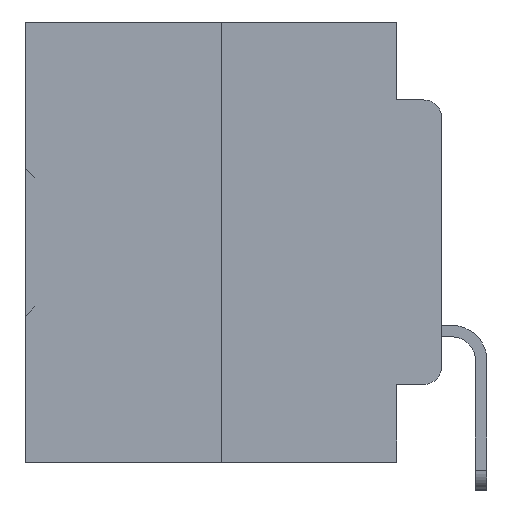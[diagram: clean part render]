
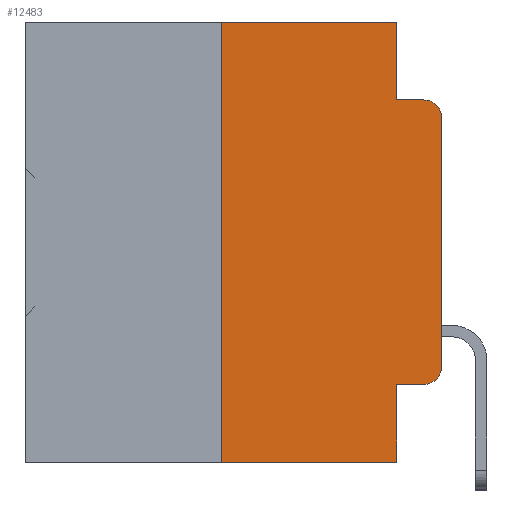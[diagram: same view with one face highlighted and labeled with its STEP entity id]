
A CAD part, left-side view. The second image highlights one B-rep face of the part: STEP entity #12483.
In plain terms, the highlighted planar face has unit normal (-1, 0, 0).
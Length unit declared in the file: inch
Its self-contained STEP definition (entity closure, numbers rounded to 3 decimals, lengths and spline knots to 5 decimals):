
#5 = VERTEX_POINT ( 'NONE', #7042 ) ;
#794 = DIRECTION ( 'NONE',  ( 0., 0., -1. ) ) ;
#1691 = LINE ( 'NONE', #23478, #37934 ) ;
#2108 = VECTOR ( 'NONE', #36460, 39.37008 ) ;
#2317 = ORIENTED_EDGE ( 'NONE', *, *, #12704, .T. ) ;
#4938 = DIRECTION ( 'NONE',  ( 0., -1., 0. ) ) ;
#5136 = ORIENTED_EDGE ( 'NONE', *, *, #24093, .F. ) ;
#5487 = CARTESIAN_POINT ( 'NONE',  ( 0., 0.051, -0.0885 ) ) ;
#5752 = CARTESIAN_POINT ( 'NONE',  ( 0., 0.051, 0. ) ) ;
#5844 = VERTEX_POINT ( 'NONE', #18852 ) ;
#5960 = CARTESIAN_POINT ( 'NONE',  ( 0., 0.25, -0.5 ) ) ;
#6009 = FACE_OUTER_BOUND ( 'NONE', #28974, .T. ) ;
#7042 = CARTESIAN_POINT ( 'NONE',  ( 0., 0.25, 0. ) ) ;
#7166 = ORIENTED_EDGE ( 'NONE', *, *, #31927, .F. ) ;
#7660 = ORIENTED_EDGE ( 'NONE', *, *, #35745, .T. ) ;
#8333 = VERTEX_POINT ( 'NONE', #28613 ) ;
#8835 = DIRECTION ( 'NONE',  ( 0., 0., 1. ) ) ;
#9024 = LINE ( 'NONE', #33836, #24628 ) ;
#9383 = LINE ( 'NONE', #26685, #24074 ) ;
#10412 = DIRECTION ( 'NONE',  ( -1., 0., 0. ) ) ;
#10685 = CIRCLE ( 'NONE', #13943, 0.02 ) ;
#10691 = CARTESIAN_POINT ( 'NONE',  ( 0., 0.473, -0.5 ) ) ;
#11314 = VERTEX_POINT ( 'NONE', #21242 ) ;
#11740 = CARTESIAN_POINT ( 'NONE',  ( 0., 0., -0.1085 ) ) ;
#12118 = DIRECTION ( 'NONE',  ( 1., 0., 0. ) ) ;
#12179 = EDGE_CURVE ( 'NONE', #37911, #8333, #18292, .T. ) ;
#12483 = ADVANCED_FACE ( 'NONE', ( #6009 ), #29368, .F. ) ;
#12704 = EDGE_CURVE ( 'NONE', #28654, #32294, #13652, .T. ) ;
#13652 = LINE ( 'NONE', #24791, #28038 ) ;
#13943 = AXIS2_PLACEMENT_3D ( 'NONE', #32713, #15621, #35581 ) ;
#14199 = VERTEX_POINT ( 'NONE', #5752 ) ;
#14559 = CARTESIAN_POINT ( 'NONE',  ( 0., 0., -0.3915 ) ) ;
#14726 = AXIS2_PLACEMENT_3D ( 'NONE', #27756, #10412, #30608 ) ;
#15190 = ORIENTED_EDGE ( 'NONE', *, *, #22421, .F. ) ;
#15415 = ORIENTED_EDGE ( 'NONE', *, *, #16649, .T. ) ;
#15621 = DIRECTION ( 'NONE',  ( -1., 0., 0. ) ) ;
#16649 = EDGE_CURVE ( 'NONE', #32294, #11314, #37932, .T. ) ;
#16724 = ORIENTED_EDGE ( 'NONE', *, *, #20498, .F. ) ;
#16985 = CARTESIAN_POINT ( 'NONE',  ( 0., 0.473, 0. ) ) ;
#18292 = LINE ( 'NONE', #10691, #2108 ) ;
#18852 = CARTESIAN_POINT ( 'NONE',  ( 0., 0.02, -0.4115 ) ) ;
#19117 = VECTOR ( 'NONE', #26207, 39.37008 ) ;
#19255 = AXIS2_PLACEMENT_3D ( 'NONE', #23676, #12118, #32208 ) ;
#20486 = CARTESIAN_POINT ( 'NONE',  ( 0., 0.051, 0. ) ) ;
#20498 = EDGE_CURVE ( 'NONE', #31706, #11314, #9024, .T. ) ;
#21242 = CARTESIAN_POINT ( 'NONE',  ( 0., 0.02, -0.0885 ) ) ;
#21889 = DIRECTION ( 'NONE',  ( 0., 0., 1. ) ) ;
#21943 = CARTESIAN_POINT ( 'NONE',  ( 0., 0.051, 0. ) ) ;
#22421 = EDGE_CURVE ( 'NONE', #14199, #31706, #26666, .T. ) ;
#22614 = ORIENTED_EDGE ( 'NONE', *, *, #12179, .T. ) ;
#23478 = CARTESIAN_POINT ( 'NONE',  ( 0., 0.25, 0. ) ) ;
#23676 = CARTESIAN_POINT ( 'NONE',  ( 0., 0.473, 0. ) ) ;
#24074 = VECTOR ( 'NONE', #29557, 39.37008 ) ;
#24093 = EDGE_CURVE ( 'NONE', #5, #14199, #32750, .T. ) ;
#24628 = VECTOR ( 'NONE', #36689, 39.37008 ) ;
#24791 = CARTESIAN_POINT ( 'NONE',  ( 0., 0., 0. ) ) ;
#25548 = ORIENTED_EDGE ( 'NONE', *, *, #33841, .T. ) ;
#26207 = DIRECTION ( 'NONE',  ( 0., 0., -1. ) ) ;
#26666 = LINE ( 'NONE', #20486, #19117 ) ;
#26685 = CARTESIAN_POINT ( 'NONE',  ( 0., 0.051, -0.4115 ) ) ;
#26774 = ORIENTED_EDGE ( 'NONE', *, *, #30031, .F. ) ;
#27756 = CARTESIAN_POINT ( 'NONE',  ( 0., 0.02, -0.1085 ) ) ;
#27915 = CARTESIAN_POINT ( 'NONE',  ( 0., 0.051, -0.4115 ) ) ;
#28038 = VECTOR ( 'NONE', #21889, 39.37008 ) ;
#28613 = CARTESIAN_POINT ( 'NONE',  ( 0., 0.051, -0.5 ) ) ;
#28654 = VERTEX_POINT ( 'NONE', #14559 ) ;
#28974 = EDGE_LOOP ( 'NONE', ( #2317, #15415, #16724, #15190, #5136, #26774, #22614, #7166, #25548, #7660 ) ) ;
#29368 = PLANE ( 'NONE',  #19255 ) ;
#29557 = DIRECTION ( 'NONE',  ( 0., -1., 0. ) ) ;
#30031 = EDGE_CURVE ( 'NONE', #37911, #5, #1691, .T. ) ;
#30072 = VECTOR ( 'NONE', #794, 39.37008 ) ;
#30608 = DIRECTION ( 'NONE',  ( 0., 0., -1. ) ) ;
#31706 = VERTEX_POINT ( 'NONE', #5487 ) ;
#31864 = VECTOR ( 'NONE', #4938, 39.37008 ) ;
#31927 = EDGE_CURVE ( 'NONE', #35298, #8333, #36737, .T. ) ;
#32208 = DIRECTION ( 'NONE',  ( 0., 0., -1. ) ) ;
#32294 = VERTEX_POINT ( 'NONE', #11740 ) ;
#32713 = CARTESIAN_POINT ( 'NONE',  ( 0., 0.02, -0.3915 ) ) ;
#32750 = LINE ( 'NONE', #16985, #31864 ) ;
#33836 = CARTESIAN_POINT ( 'NONE',  ( 0., 0.051, -0.0885 ) ) ;
#33841 = EDGE_CURVE ( 'NONE', #35298, #5844, #9383, .T. ) ;
#35298 = VERTEX_POINT ( 'NONE', #27915 ) ;
#35581 = DIRECTION ( 'NONE',  ( 0., 0., -1. ) ) ;
#35745 = EDGE_CURVE ( 'NONE', #5844, #28654, #10685, .T. ) ;
#36460 = DIRECTION ( 'NONE',  ( 0., -1., 0. ) ) ;
#36689 = DIRECTION ( 'NONE',  ( 0., -1., 0. ) ) ;
#36737 = LINE ( 'NONE', #21943, #30072 ) ;
#37911 = VERTEX_POINT ( 'NONE', #5960 ) ;
#37932 = CIRCLE ( 'NONE', #14726, 0.02 ) ;
#37934 = VECTOR ( 'NONE', #8835, 39.37008 ) ;
